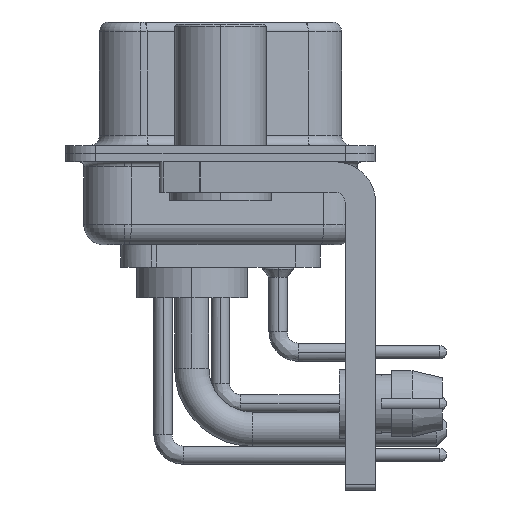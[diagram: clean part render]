
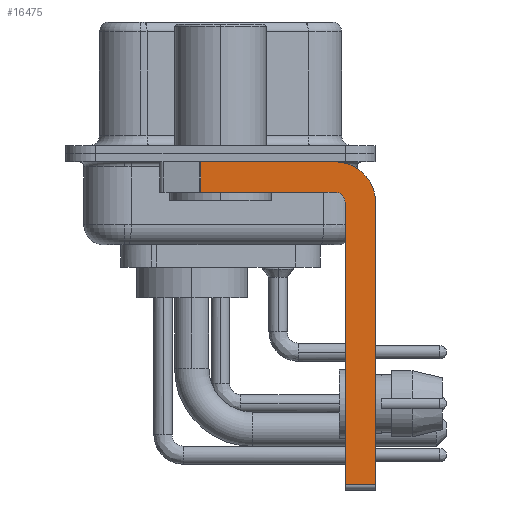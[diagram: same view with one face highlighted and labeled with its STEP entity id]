
A CAD part, left-side view. The second image highlights one B-rep face of the part: STEP entity #16475.
In plain terms, the highlighted planar face has unit normal (-1, 0, 0).
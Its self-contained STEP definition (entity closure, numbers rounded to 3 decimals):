
#27 = LINE ( 'NONE', #29736, #10509 ) ;
#136 = ORIENTED_EDGE ( 'NONE', *, *, #23686, .F. ) ;
#458 = AXIS2_PLACEMENT_3D ( 'NONE', #17757, #3719, #27411 ) ;
#845 = ORIENTED_EDGE ( 'NONE', *, *, #2240, .F. ) ;
#1690 = CIRCLE ( 'NONE', #458, 0.5 ) ;
#1853 = DIRECTION ( 'NONE',  ( 1., 0., 0. ) ) ;
#2061 = LINE ( 'NONE', #26988, #21486 ) ;
#2240 = EDGE_CURVE ( 'NONE', #28489, #34219, #3752, .T. ) ;
#3719 = DIRECTION ( 'NONE',  ( -1., 0., 0. ) ) ;
#3752 = CIRCLE ( 'NONE', #4375, 2. ) ;
#4375 = AXIS2_PLACEMENT_3D ( 'NONE', #11180, #1853, #11374 ) ;
#4616 = VECTOR ( 'NONE', #23373, 1000. ) ;
#5044 = VERTEX_POINT ( 'NONE', #14199 ) ;
#5925 = CARTESIAN_POINT ( 'NONE',  ( -2.9, -5.65, -2.4 ) ) ;
#6132 = VERTEX_POINT ( 'NONE', #33213 ) ;
#6244 = DIRECTION ( 'NONE',  ( 0., -1., 0. ) ) ;
#6341 = CARTESIAN_POINT ( 'NONE',  ( -2.9, -5.65, -16.35 ) ) ;
#6568 = VERTEX_POINT ( 'NONE', #24070 ) ;
#7198 = ORIENTED_EDGE ( 'NONE', *, *, #15666, .F. ) ;
#7262 = EDGE_CURVE ( 'NONE', #6568, #28489, #27, .T. ) ;
#8257 = EDGE_CURVE ( 'NONE', #9130, #24514, #17991, .T. ) ;
#8653 = DIRECTION ( 'NONE',  ( 0., 0., -1. ) ) ;
#9130 = VERTEX_POINT ( 'NONE', #11501 ) ;
#9228 = PLANE ( 'NONE',  #15335 ) ;
#10119 = CARTESIAN_POINT ( 'NONE',  ( -2.9, -5.65, -0.4 ) ) ;
#10509 = VECTOR ( 'NONE', #6244, 1000. ) ;
#10783 = ORIENTED_EDGE ( 'NONE', *, *, #8257, .T. ) ;
#11180 = CARTESIAN_POINT ( 'NONE',  ( -2.9, -5.65, -2.4 ) ) ;
#11374 = DIRECTION ( 'NONE',  ( 0., 0., -1. ) ) ;
#11501 = CARTESIAN_POINT ( 'NONE',  ( -2.9, -6.15, -16.35 ) ) ;
#11627 = ORIENTED_EDGE ( 'NONE', *, *, #18268, .F. ) ;
#11947 = DIRECTION ( 'NONE',  ( 1., 0., 0. ) ) ;
#14199 = CARTESIAN_POINT ( 'NONE',  ( -2.9, 0.978, -1.9 ) ) ;
#14422 = LINE ( 'NONE', #23183, #4616 ) ;
#15335 = AXIS2_PLACEMENT_3D ( 'NONE', #5925, #11947, #8653 ) ;
#15666 = EDGE_CURVE ( 'NONE', #23568, #5044, #2061, .T. ) ;
#16475 = ADVANCED_FACE ( 'NONE', ( #38315 ), #9228, .F. ) ;
#17757 = CARTESIAN_POINT ( 'NONE',  ( -2.9, -5.65, -2.4 ) ) ;
#17991 = LINE ( 'NONE', #6341, #21751 ) ;
#18268 = EDGE_CURVE ( 'NONE', #34219, #24514, #14422, .T. ) ;
#19483 = EDGE_CURVE ( 'NONE', #6568, #5044, #27668, .T. ) ;
#19900 = ORIENTED_EDGE ( 'NONE', *, *, #19483, .T. ) ;
#21124 = EDGE_CURVE ( 'NONE', #9130, #6132, #38274, .T. ) ;
#21486 = VECTOR ( 'NONE', #32993, 1000. ) ;
#21751 = VECTOR ( 'NONE', #33511, 1000. ) ;
#22979 = DIRECTION ( 'NONE',  ( 0., 0., 1. ) ) ;
#23183 = CARTESIAN_POINT ( 'NONE',  ( -2.9, -7.65, -2.4 ) ) ;
#23373 = DIRECTION ( 'NONE',  ( 0., 0., -1. ) ) ;
#23568 = VERTEX_POINT ( 'NONE', #26301 ) ;
#23671 = ORIENTED_EDGE ( 'NONE', *, *, #7262, .F. ) ;
#23686 = EDGE_CURVE ( 'NONE', #6132, #23568, #1690, .T. ) ;
#24070 = CARTESIAN_POINT ( 'NONE',  ( -2.9, 0.978, -0.4 ) ) ;
#24514 = VERTEX_POINT ( 'NONE', #30329 ) ;
#26301 = CARTESIAN_POINT ( 'NONE',  ( -2.9, -5.65, -1.9 ) ) ;
#26770 = ORIENTED_EDGE ( 'NONE', *, *, #21124, .F. ) ;
#26988 = CARTESIAN_POINT ( 'NONE',  ( -2.9, -5.65, -1.9 ) ) ;
#27411 = DIRECTION ( 'NONE',  ( 0., 0., 1. ) ) ;
#27570 = CARTESIAN_POINT ( 'NONE',  ( -2.9, -7.65, -2.4 ) ) ;
#27668 = LINE ( 'NONE', #32892, #30647 ) ;
#28489 = VERTEX_POINT ( 'NONE', #10119 ) ;
#29736 = CARTESIAN_POINT ( 'NONE',  ( -2.9, 3., -0.4 ) ) ;
#30183 = DIRECTION ( 'NONE',  ( 0., 0., -1. ) ) ;
#30329 = CARTESIAN_POINT ( 'NONE',  ( -2.9, -7.65, -16.35 ) ) ;
#30647 = VECTOR ( 'NONE', #30183, 1000. ) ;
#31889 = CARTESIAN_POINT ( 'NONE',  ( -2.9, -6.15, -16.6 ) ) ;
#32892 = CARTESIAN_POINT ( 'NONE',  ( -2.9, 0.978, -1.9 ) ) ;
#32993 = DIRECTION ( 'NONE',  ( 0., 1., 0. ) ) ;
#33213 = CARTESIAN_POINT ( 'NONE',  ( -2.9, -6.15, -2.4 ) ) ;
#33511 = DIRECTION ( 'NONE',  ( 0., -1., 0. ) ) ;
#34219 = VERTEX_POINT ( 'NONE', #27570 ) ;
#36250 = EDGE_LOOP ( 'NONE', ( #23671, #19900, #7198, #136, #26770, #10783, #11627, #845 ) ) ;
#36935 = VECTOR ( 'NONE', #22979, 1000. ) ;
#38274 = LINE ( 'NONE', #31889, #36935 ) ;
#38315 = FACE_OUTER_BOUND ( 'NONE', #36250, .T. ) ;
